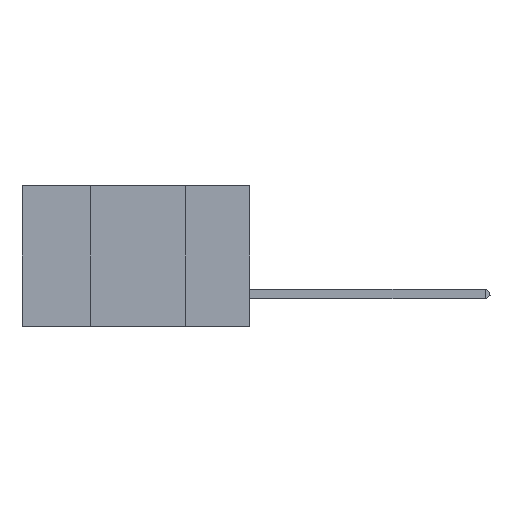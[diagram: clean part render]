
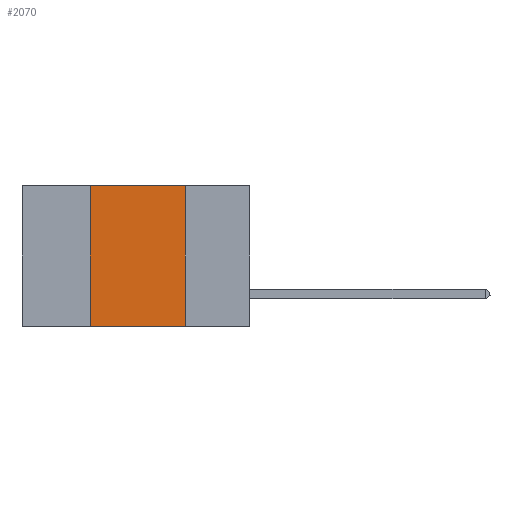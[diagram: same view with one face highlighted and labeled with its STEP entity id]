
A CAD part, left-side view. The second image highlights one B-rep face of the part: STEP entity #2070.
In plain terms, the highlighted planar face has unit normal (-1, 0, 0).
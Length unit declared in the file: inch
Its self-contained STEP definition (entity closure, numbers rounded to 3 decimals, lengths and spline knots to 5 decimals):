
#23 = EDGE_CURVE ( 'NONE', #3755, #24979, #34212, .T. ) ;
#785 = ORIENTED_EDGE ( 'NONE', *, *, #23, .F. ) ;
#1232 = VERTEX_POINT ( 'NONE', #25102 ) ;
#2070 = ADVANCED_FACE ( 'NONE', ( #36055 ), #19793, .F. ) ;
#2230 = DIRECTION ( 'NONE',  ( 0., 0., -1. ) ) ;
#2611 = VECTOR ( 'NONE', #2230, 39.37008 ) ;
#3755 = VERTEX_POINT ( 'NONE', #21316 ) ;
#3982 = LINE ( 'NONE', #21067, #45029 ) ;
#6312 = ORIENTED_EDGE ( 'NONE', *, *, #24963, .T. ) ;
#9592 = CARTESIAN_POINT ( 'NONE',  ( 0., 0.42, 0. ) ) ;
#10394 = ORIENTED_EDGE ( 'NONE', *, *, #44258, .F. ) ;
#12829 = CARTESIAN_POINT ( 'NONE',  ( 0., 0.6, -0.37 ) ) ;
#13178 = DIRECTION ( 'NONE',  ( 0., 0., 1. ) ) ;
#15179 = EDGE_LOOP ( 'NONE', ( #785, #10394, #17833, #6312 ) ) ;
#17833 = ORIENTED_EDGE ( 'NONE', *, *, #26326, .F. ) ;
#19793 = PLANE ( 'NONE',  #42764 ) ;
#19936 = CARTESIAN_POINT ( 'NONE',  ( 0., 0.6, 0. ) ) ;
#20406 = VECTOR ( 'NONE', #37553, 39.37008 ) ;
#21067 = CARTESIAN_POINT ( 'NONE',  ( 0., 0.6, 0. ) ) ;
#21316 = CARTESIAN_POINT ( 'NONE',  ( 0., 0.17, 0. ) ) ;
#21363 = DIRECTION ( 'NONE',  ( 0., -1., 0. ) ) ;
#23879 = LINE ( 'NONE', #9592, #36627 ) ;
#24083 = VERTEX_POINT ( 'NONE', #31111 ) ;
#24963 = EDGE_CURVE ( 'NONE', #1232, #24979, #26476, .T. ) ;
#24979 = VERTEX_POINT ( 'NONE', #45457 ) ;
#25102 = CARTESIAN_POINT ( 'NONE',  ( 0., 0.42, -0.37 ) ) ;
#26326 = EDGE_CURVE ( 'NONE', #1232, #24083, #23879, .T. ) ;
#26476 = LINE ( 'NONE', #12829, #20406 ) ;
#30146 = DIRECTION ( 'NONE',  ( 1., 0., 0. ) ) ;
#31111 = CARTESIAN_POINT ( 'NONE',  ( 0., 0.42, 0. ) ) ;
#33422 = DIRECTION ( 'NONE',  ( 0., 0., -1. ) ) ;
#34212 = LINE ( 'NONE', #41091, #2611 ) ;
#36055 = FACE_OUTER_BOUND ( 'NONE', #15179, .T. ) ;
#36627 = VECTOR ( 'NONE', #13178, 39.37008 ) ;
#37553 = DIRECTION ( 'NONE',  ( 0., -1., 0. ) ) ;
#41091 = CARTESIAN_POINT ( 'NONE',  ( 0., 0.17, 0. ) ) ;
#42764 = AXIS2_PLACEMENT_3D ( 'NONE', #19936, #30146, #33422 ) ;
#44258 = EDGE_CURVE ( 'NONE', #24083, #3755, #3982, .T. ) ;
#45029 = VECTOR ( 'NONE', #21363, 39.37008 ) ;
#45457 = CARTESIAN_POINT ( 'NONE',  ( 0., 0.17, -0.37 ) ) ;
